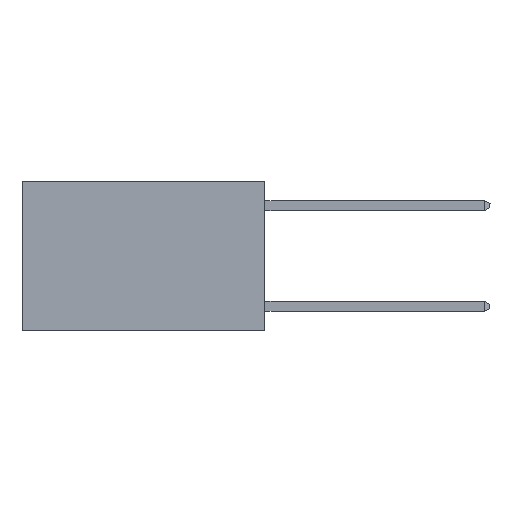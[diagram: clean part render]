
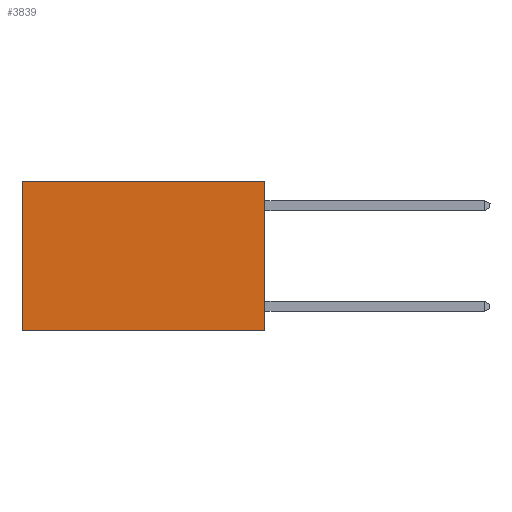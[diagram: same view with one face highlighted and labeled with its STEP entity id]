
A CAD part, left-side view. The second image highlights one B-rep face of the part: STEP entity #3839.
In plain terms, the highlighted planar face has unit normal (-1, 0, 0).
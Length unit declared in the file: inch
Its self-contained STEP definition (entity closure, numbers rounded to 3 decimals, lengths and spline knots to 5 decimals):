
#207 = VECTOR ( 'NONE', #5223, 39.37008 ) ;
#218 = ORIENTED_EDGE ( 'NONE', *, *, #5148, .F. ) ;
#242 = ORIENTED_EDGE ( 'NONE', *, *, #28222, .F. ) ;
#838 = CARTESIAN_POINT ( 'NONE',  ( 0.2625, 0.6, 0. ) ) ;
#1113 = DIRECTION ( 'NONE',  ( 1., 0., 0. ) ) ;
#2032 = LINE ( 'NONE', #6952, #28121 ) ;
#2055 = VERTEX_POINT ( 'NONE', #838 ) ;
#3839 = ADVANCED_FACE ( 'NONE', ( #19668 ), #17249, .F. ) ;
#3996 = ORIENTED_EDGE ( 'NONE', *, *, #26343, .T. ) ;
#5148 = EDGE_CURVE ( 'NONE', #13818, #24679, #11760, .T. ) ;
#5223 = DIRECTION ( 'NONE',  ( 0., 0., -1. ) ) ;
#5537 = VECTOR ( 'NONE', #22878, 39.37008 ) ;
#6353 = VERTEX_POINT ( 'NONE', #11173 ) ;
#6952 = CARTESIAN_POINT ( 'NONE',  ( 0.2625, 0., 0. ) ) ;
#7170 = EDGE_LOOP ( 'NONE', ( #17396, #218, #242, #3996 ) ) ;
#7524 = LINE ( 'NONE', #12292, #207 ) ;
#8545 = CARTESIAN_POINT ( 'NONE',  ( 0.2625, 0., -0.37 ) ) ;
#11173 = CARTESIAN_POINT ( 'NONE',  ( 0.2625, 0., 0. ) ) ;
#11760 = LINE ( 'NONE', #16494, #21312 ) ;
#12292 = CARTESIAN_POINT ( 'NONE',  ( 0.2625, 0., 0. ) ) ;
#12447 = EDGE_CURVE ( 'NONE', #2055, #24679, #27009, .T. ) ;
#13818 = VERTEX_POINT ( 'NONE', #8545 ) ;
#14060 = DIRECTION ( 'NONE',  ( 0., 1., 0. ) ) ;
#16494 = CARTESIAN_POINT ( 'NONE',  ( 0.2625, 0., -0.37 ) ) ;
#17249 = PLANE ( 'NONE',  #27620 ) ;
#17396 = ORIENTED_EDGE ( 'NONE', *, *, #12447, .T. ) ;
#17397 = CARTESIAN_POINT ( 'NONE',  ( 0.2625, 0., 0. ) ) ;
#19130 = CARTESIAN_POINT ( 'NONE',  ( 0.2625, 0.6, 0. ) ) ;
#19668 = FACE_OUTER_BOUND ( 'NONE', #7170, .T. ) ;
#21312 = VECTOR ( 'NONE', #14060, 39.37008 ) ;
#22878 = DIRECTION ( 'NONE',  ( 0., 0., -1. ) ) ;
#23798 = CARTESIAN_POINT ( 'NONE',  ( 0.2625, 0.6, -0.37 ) ) ;
#24679 = VERTEX_POINT ( 'NONE', #23798 ) ;
#26343 = EDGE_CURVE ( 'NONE', #6353, #2055, #2032, .T. ) ;
#27009 = LINE ( 'NONE', #19130, #5537 ) ;
#27620 = AXIS2_PLACEMENT_3D ( 'NONE', #17397, #1113, #28879 ) ;
#27946 = DIRECTION ( 'NONE',  ( 0., 1., 0. ) ) ;
#28121 = VECTOR ( 'NONE', #27946, 39.37008 ) ;
#28222 = EDGE_CURVE ( 'NONE', #6353, #13818, #7524, .T. ) ;
#28879 = DIRECTION ( 'NONE',  ( 0., 0., -1. ) ) ;
